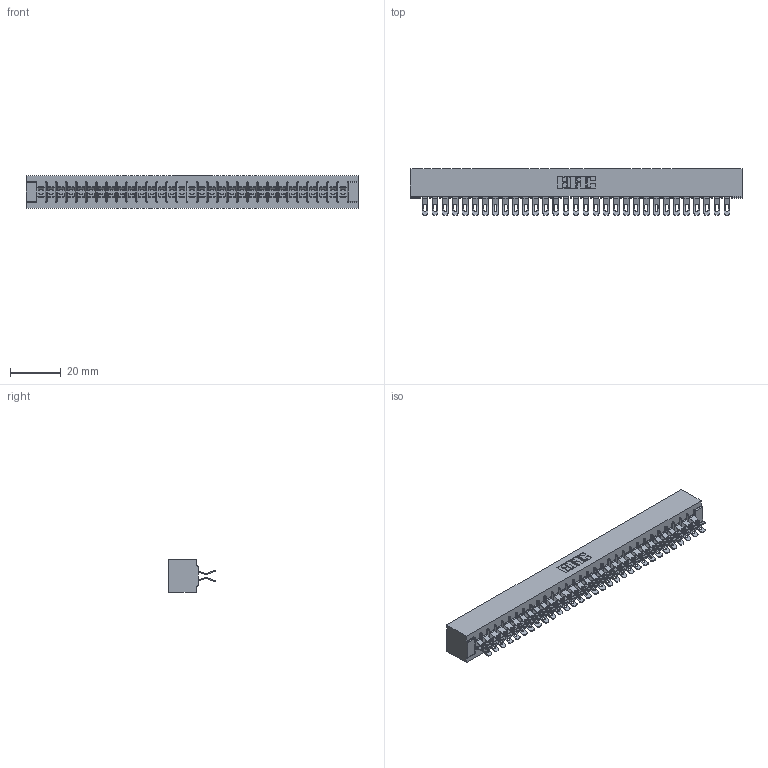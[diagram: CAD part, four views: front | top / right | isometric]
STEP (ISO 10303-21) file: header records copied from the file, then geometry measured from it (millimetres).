
FILE_DESCRIPTION (( 'STEP AP203' ), '1' );
FILE_NAME ('315-062-555-201.STEP', '2019-09-10T20:18:40', ( '' ), ( '' ), 'SwSTEP 2.0', 'SolidWorks 2016', '' );
FILE_SCHEMA (( 'CONFIG_CONTROL_DESIGN' ));
Length unit declared in the file: inch
Products named in the file (3): 305-290-001_555; 315-062-555-201; 305 Part_No Mounting
Assembly tree (63 placements, depth 2):
  315-062-555-201
    305 Part_No Mounting
    305-290-001_555  x62
Bounding box: 130.71 x 18.41 x 12.7 mm (x, y, z)
Volume: 14241.4 mm3; surface area: 19431.2 mm2
Topology: 63 solids, 63 shells, 4200 faces, 12537 edges, 8190 vertices
Faces by surface type: plane 2048, cylinder 2028, sphere 124
Entity records: 35250 total; most frequent: CARTESIAN_POINT 5849, ORIENTED_EDGE 5794, DIRECTION 5659, EDGE_CURVE 2897, LINE 2315, VECTOR 2315, VERTEX_POINT 1846, AXIS2_PLACEMENT_3D 1672
